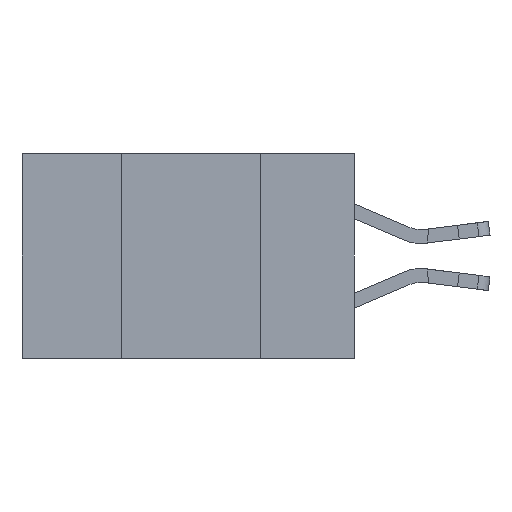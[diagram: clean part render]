
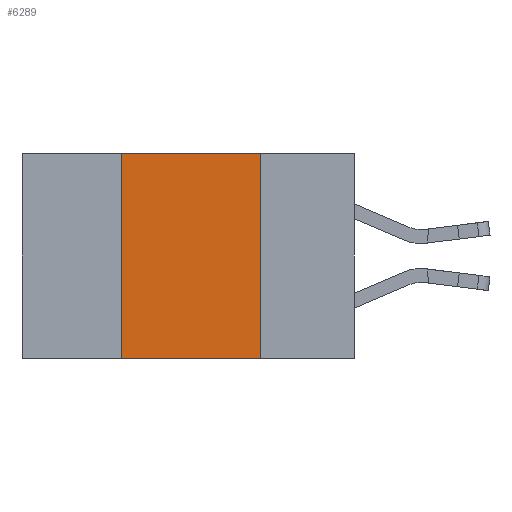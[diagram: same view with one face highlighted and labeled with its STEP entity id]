
A CAD part, left-side view. The second image highlights one B-rep face of the part: STEP entity #6289.
In plain terms, the highlighted planar face has unit normal (-1, 0, 0).
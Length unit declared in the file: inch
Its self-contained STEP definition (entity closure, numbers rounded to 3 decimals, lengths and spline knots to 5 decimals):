
#32 = CARTESIAN_POINT ( 'NONE',  ( 0., 0.6, 0. ) ) ;
#124 = DIRECTION ( 'NONE',  ( 0., 0., -1. ) ) ;
#300 = DIRECTION ( 'NONE',  ( 0., -1., 0. ) ) ;
#371 = ORIENTED_EDGE ( 'NONE', *, *, #17379, .F. ) ;
#389 = EDGE_CURVE ( 'NONE', #805, #2357, #11467, .T. ) ;
#805 = VERTEX_POINT ( 'NONE', #14148 ) ;
#834 = EDGE_CURVE ( 'NONE', #8903, #2357, #10230, .T. ) ;
#1688 = CARTESIAN_POINT ( 'NONE',  ( 0., 0.17, -0.37 ) ) ;
#1709 = ORIENTED_EDGE ( 'NONE', *, *, #389, .F. ) ;
#1816 = FACE_OUTER_BOUND ( 'NONE', #4108, .T. ) ;
#2357 = VERTEX_POINT ( 'NONE', #10169 ) ;
#2755 = CARTESIAN_POINT ( 'NONE',  ( 0., 0.42, -0.37 ) ) ;
#3554 = ORIENTED_EDGE ( 'NONE', *, *, #12666, .F. ) ;
#3657 = DIRECTION ( 'NONE',  ( 1., 0., 0. ) ) ;
#4108 = EDGE_LOOP ( 'NONE', ( #1709, #371, #3554, #10214 ) ) ;
#4298 = LINE ( 'NONE', #32, #16303 ) ;
#5358 = VERTEX_POINT ( 'NONE', #12571 ) ;
#5817 = LINE ( 'NONE', #2755, #15011 ) ;
#6289 = ADVANCED_FACE ( 'NONE', ( #1816 ), #16644, .F. ) ;
#6378 = CARTESIAN_POINT ( 'NONE',  ( 0., 0.6, 0. ) ) ;
#7549 = AXIS2_PLACEMENT_3D ( 'NONE', #6378, #3657, #17873 ) ;
#8598 = VECTOR ( 'NONE', #10325, 39.37008 ) ;
#8903 = VERTEX_POINT ( 'NONE', #11852 ) ;
#10169 = CARTESIAN_POINT ( 'NONE',  ( 0., 0.17, -0.37 ) ) ;
#10214 = ORIENTED_EDGE ( 'NONE', *, *, #834, .T. ) ;
#10230 = LINE ( 'NONE', #14239, #8598 ) ;
#10325 = DIRECTION ( 'NONE',  ( 0., -1., 0. ) ) ;
#11410 = DIRECTION ( 'NONE',  ( 0., 0., 1. ) ) ;
#11467 = LINE ( 'NONE', #1688, #16020 ) ;
#11852 = CARTESIAN_POINT ( 'NONE',  ( 0., 0.42, -0.37 ) ) ;
#12571 = CARTESIAN_POINT ( 'NONE',  ( 0., 0.42, 0. ) ) ;
#12666 = EDGE_CURVE ( 'NONE', #8903, #5358, #5817, .T. ) ;
#14148 = CARTESIAN_POINT ( 'NONE',  ( 0., 0.17, 0. ) ) ;
#14239 = CARTESIAN_POINT ( 'NONE',  ( 0., 0.6, -0.37 ) ) ;
#15011 = VECTOR ( 'NONE', #11410, 39.37008 ) ;
#16020 = VECTOR ( 'NONE', #124, 39.37008 ) ;
#16303 = VECTOR ( 'NONE', #300, 39.37008 ) ;
#16644 = PLANE ( 'NONE',  #7549 ) ;
#17379 = EDGE_CURVE ( 'NONE', #5358, #805, #4298, .T. ) ;
#17873 = DIRECTION ( 'NONE',  ( 0., 0., -1. ) ) ;
